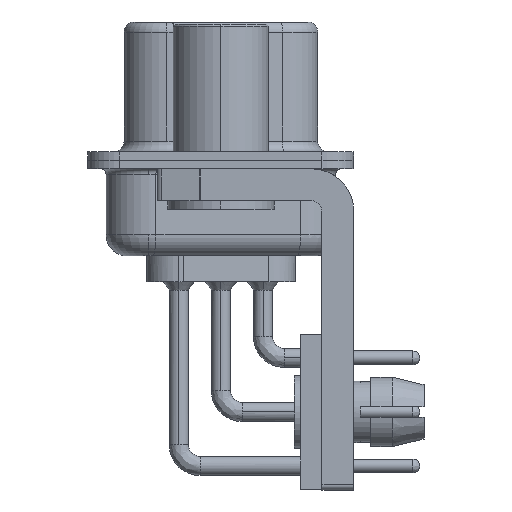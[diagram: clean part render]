
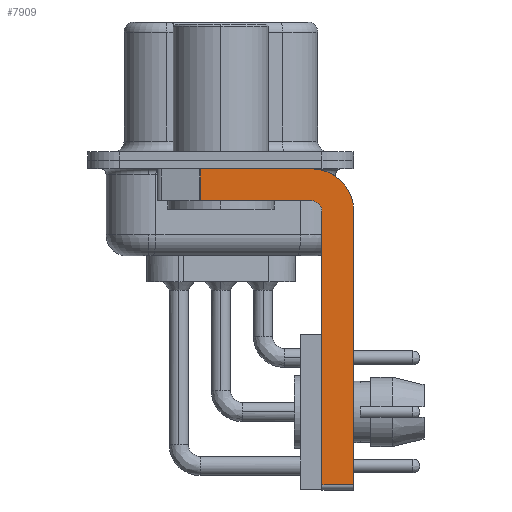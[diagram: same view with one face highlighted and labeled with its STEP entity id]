
A CAD part, left-side view. The second image highlights one B-rep face of the part: STEP entity #7909.
In plain terms, the highlighted planar face has unit normal (-1, 0, 0).
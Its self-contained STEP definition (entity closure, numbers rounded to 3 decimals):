
#31 = VERTEX_POINT ( 'NONE', #18047 ) ;
#211 = VECTOR ( 'NONE', #24874, 1000. ) ;
#992 = LINE ( 'NONE', #22077, #34143 ) ;
#2996 = DIRECTION ( 'NONE',  ( 0., 0., -1. ) ) ;
#4056 = CARTESIAN_POINT ( 'NONE',  ( -2.9, -6.25, -2.4 ) ) ;
#4557 = DIRECTION ( 'NONE',  ( 0., 0., -1. ) ) ;
#5633 = CARTESIAN_POINT ( 'NONE',  ( -2.9, -4.75, -15.5 ) ) ;
#6183 = VECTOR ( 'NONE', #2996, 1000. ) ;
#6689 = DIRECTION ( 'NONE',  ( 0., -1., 0. ) ) ;
#7691 = ORIENTED_EDGE ( 'NONE', *, *, #29538, .F. ) ;
#7823 = VECTOR ( 'NONE', #13116, 1000. ) ;
#7909 = ADVANCED_FACE ( 'NONE', ( #13349 ), #39803, .F. ) ;
#7979 = VERTEX_POINT ( 'NONE', #27275 ) ;
#10383 = DIRECTION ( 'NONE',  ( 1., 0., 0. ) ) ;
#13116 = DIRECTION ( 'NONE',  ( 0., 1., 0. ) ) ;
#13349 = FACE_OUTER_BOUND ( 'NONE', #16730, .T. ) ;
#15270 = AXIS2_PLACEMENT_3D ( 'NONE', #37953, #18674, #41217 ) ;
#15433 = EDGE_CURVE ( 'NONE', #7979, #19926, #19219, .T. ) ;
#16219 = VERTEX_POINT ( 'NONE', #23634 ) ;
#16455 = ORIENTED_EDGE ( 'NONE', *, *, #39219, .F. ) ;
#16730 = EDGE_LOOP ( 'NONE', ( #16968, #26987, #27944, #7691, #25272, #27791, #16455, #26881 ) ) ;
#16968 = ORIENTED_EDGE ( 'NONE', *, *, #15433, .F. ) ;
#18047 = CARTESIAN_POINT ( 'NONE',  ( -2.9, -6.25, -15.25 ) ) ;
#18141 = EDGE_CURVE ( 'NONE', #7979, #36218, #32786, .T. ) ;
#18190 = VECTOR ( 'NONE', #6689, 1000. ) ;
#18674 = DIRECTION ( 'NONE',  ( -1., 0., 0. ) ) ;
#19172 = CARTESIAN_POINT ( 'NONE',  ( -2.9, -4.25, -1.9 ) ) ;
#19219 = LINE ( 'NONE', #38684, #18190 ) ;
#19302 = VERTEX_POINT ( 'NONE', #31702 ) ;
#19832 = CIRCLE ( 'NONE', #28950, 2. ) ;
#19926 = VERTEX_POINT ( 'NONE', #41501 ) ;
#20546 = CARTESIAN_POINT ( 'NONE',  ( -2.9, -4.25, -2.4 ) ) ;
#22077 = CARTESIAN_POINT ( 'NONE',  ( -2.9, -4.25, -15.25 ) ) ;
#22860 = CARTESIAN_POINT ( 'NONE',  ( -2.9, 0.978, -1.9 ) ) ;
#23146 = DIRECTION ( 'NONE',  ( 0., 0., -1. ) ) ;
#23189 = CARTESIAN_POINT ( 'NONE',  ( -2.9, -4.75, -2.4 ) ) ;
#23634 = CARTESIAN_POINT ( 'NONE',  ( -2.9, -4.75, -15.25 ) ) ;
#23789 = DIRECTION ( 'NONE',  ( 1., 0., 0. ) ) ;
#24715 = EDGE_CURVE ( 'NONE', #16219, #31, #992, .T. ) ;
#24874 = DIRECTION ( 'NONE',  ( 0., 0., 1. ) ) ;
#25272 = ORIENTED_EDGE ( 'NONE', *, *, #27519, .F. ) ;
#25431 = AXIS2_PLACEMENT_3D ( 'NONE', #20546, #23789, #4557 ) ;
#26427 = VECTOR ( 'NONE', #23146, 1000. ) ;
#26881 = ORIENTED_EDGE ( 'NONE', *, *, #27176, .F. ) ;
#26987 = ORIENTED_EDGE ( 'NONE', *, *, #18141, .T. ) ;
#27176 = EDGE_CURVE ( 'NONE', #19926, #19302, #19832, .T. ) ;
#27275 = CARTESIAN_POINT ( 'NONE',  ( -2.9, 0.978, -0.4 ) ) ;
#27519 = EDGE_CURVE ( 'NONE', #16219, #29774, #33380, .T. ) ;
#27791 = ORIENTED_EDGE ( 'NONE', *, *, #24715, .T. ) ;
#27944 = ORIENTED_EDGE ( 'NONE', *, *, #30787, .F. ) ;
#28434 = LINE ( 'NONE', #4056, #26427 ) ;
#28950 = AXIS2_PLACEMENT_3D ( 'NONE', #29678, #10383, #32874 ) ;
#29538 = EDGE_CURVE ( 'NONE', #29774, #33355, #37244, .T. ) ;
#29678 = CARTESIAN_POINT ( 'NONE',  ( -2.9, -4.25, -2.4 ) ) ;
#29774 = VERTEX_POINT ( 'NONE', #23189 ) ;
#30787 = EDGE_CURVE ( 'NONE', #33355, #36218, #33432, .T. ) ;
#31702 = CARTESIAN_POINT ( 'NONE',  ( -2.9, -6.25, -2.4 ) ) ;
#32391 = CARTESIAN_POINT ( 'NONE',  ( -2.9, -4.25, -1.9 ) ) ;
#32786 = LINE ( 'NONE', #41494, #6183 ) ;
#32874 = DIRECTION ( 'NONE',  ( 0., 0., -1. ) ) ;
#33355 = VERTEX_POINT ( 'NONE', #19172 ) ;
#33380 = LINE ( 'NONE', #5633, #211 ) ;
#33432 = LINE ( 'NONE', #32391, #7823 ) ;
#34143 = VECTOR ( 'NONE', #34982, 1000. ) ;
#34982 = DIRECTION ( 'NONE',  ( 0., -1., 0. ) ) ;
#36218 = VERTEX_POINT ( 'NONE', #22860 ) ;
#37244 = CIRCLE ( 'NONE', #15270, 0.5 ) ;
#37953 = CARTESIAN_POINT ( 'NONE',  ( -2.9, -4.25, -2.4 ) ) ;
#38684 = CARTESIAN_POINT ( 'NONE',  ( -2.9, 3., -0.4 ) ) ;
#39219 = EDGE_CURVE ( 'NONE', #19302, #31, #28434, .T. ) ;
#39803 = PLANE ( 'NONE',  #25431 ) ;
#41217 = DIRECTION ( 'NONE',  ( 0., 0., 1. ) ) ;
#41494 = CARTESIAN_POINT ( 'NONE',  ( -2.9, 0.978, -1.9 ) ) ;
#41501 = CARTESIAN_POINT ( 'NONE',  ( -2.9, -4.25, -0.4 ) ) ;
